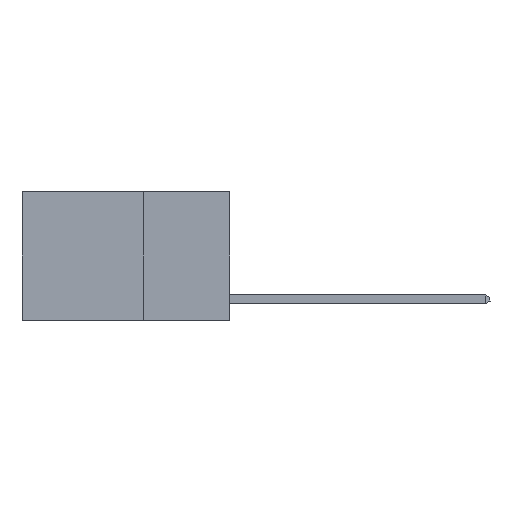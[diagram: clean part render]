
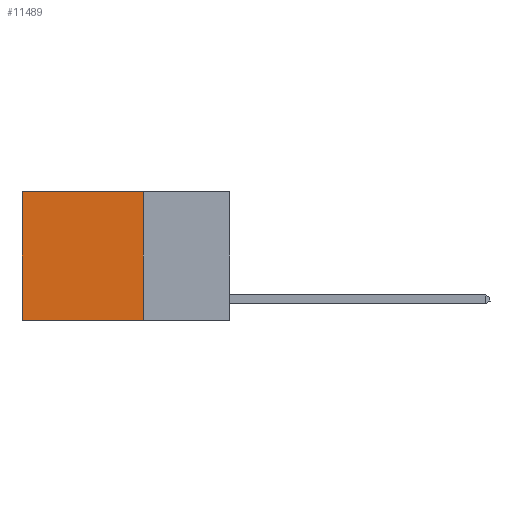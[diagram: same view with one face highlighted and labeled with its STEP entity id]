
A CAD part, left-side view. The second image highlights one B-rep face of the part: STEP entity #11489.
In plain terms, the highlighted planar face has unit normal (-1, 0, 0).
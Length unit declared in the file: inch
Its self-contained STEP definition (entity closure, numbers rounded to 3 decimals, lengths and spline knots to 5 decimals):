
#637 = DIRECTION ( 'NONE',  ( 0., 1., 0. ) ) ;
#1539 = LINE ( 'NONE', #21498, #15861 ) ;
#1577 = CARTESIAN_POINT ( 'NONE',  ( 0.2625, 0.25, 0. ) ) ;
#2979 = VECTOR ( 'NONE', #637, 39.37008 ) ;
#3474 = LINE ( 'NONE', #1577, #17716 ) ;
#3797 = LINE ( 'NONE', #17367, #2979 ) ;
#4476 = EDGE_CURVE ( 'NONE', #22231, #20335, #3797, .T. ) ;
#5365 = ORIENTED_EDGE ( 'NONE', *, *, #4476, .T. ) ;
#5876 = LINE ( 'NONE', #6581, #20098 ) ;
#6581 = CARTESIAN_POINT ( 'NONE',  ( 0.2625, 0.6, 0. ) ) ;
#6658 = VERTEX_POINT ( 'NONE', #21908 ) ;
#6901 = CARTESIAN_POINT ( 'NONE',  ( 0.2625, 0.25, 0. ) ) ;
#7337 = EDGE_CURVE ( 'NONE', #6658, #15682, #1539, .T. ) ;
#8527 = DIRECTION ( 'NONE',  ( 0., 0., -1. ) ) ;
#8565 = CARTESIAN_POINT ( 'NONE',  ( 0.2625, 0.25, 0. ) ) ;
#8723 = CARTESIAN_POINT ( 'NONE',  ( 0.2625, 0.6, -0.37 ) ) ;
#10473 = DIRECTION ( 'NONE',  ( 0., 0., -1. ) ) ;
#11489 = ADVANCED_FACE ( 'NONE', ( #19168 ), #19622, .F. ) ;
#12410 = EDGE_LOOP ( 'NONE', ( #13685, #23657, #14882, #5365 ) ) ;
#12976 = EDGE_CURVE ( 'NONE', #22231, #6658, #3474, .T. ) ;
#13608 = AXIS2_PLACEMENT_3D ( 'NONE', #8565, #21368, #10473 ) ;
#13685 = ORIENTED_EDGE ( 'NONE', *, *, #16408, .T. ) ;
#14882 = ORIENTED_EDGE ( 'NONE', *, *, #12976, .F. ) ;
#15682 = VERTEX_POINT ( 'NONE', #8723 ) ;
#15861 = VECTOR ( 'NONE', #16294, 39.37008 ) ;
#16294 = DIRECTION ( 'NONE',  ( 0., 1., 0. ) ) ;
#16408 = EDGE_CURVE ( 'NONE', #20335, #15682, #5876, .T. ) ;
#16472 = DIRECTION ( 'NONE',  ( 0., 0., -1. ) ) ;
#17367 = CARTESIAN_POINT ( 'NONE',  ( 0.2625, 0.25, 0. ) ) ;
#17716 = VECTOR ( 'NONE', #16472, 39.37008 ) ;
#19168 = FACE_OUTER_BOUND ( 'NONE', #12410, .T. ) ;
#19622 = PLANE ( 'NONE',  #13608 ) ;
#20098 = VECTOR ( 'NONE', #8527, 39.37008 ) ;
#20335 = VERTEX_POINT ( 'NONE', #23156 ) ;
#21368 = DIRECTION ( 'NONE',  ( 1., 0., 0. ) ) ;
#21498 = CARTESIAN_POINT ( 'NONE',  ( 0.2625, 0.25, -0.37 ) ) ;
#21908 = CARTESIAN_POINT ( 'NONE',  ( 0.2625, 0.25, -0.37 ) ) ;
#22231 = VERTEX_POINT ( 'NONE', #6901 ) ;
#23156 = CARTESIAN_POINT ( 'NONE',  ( 0.2625, 0.6, 0. ) ) ;
#23657 = ORIENTED_EDGE ( 'NONE', *, *, #7337, .F. ) ;
